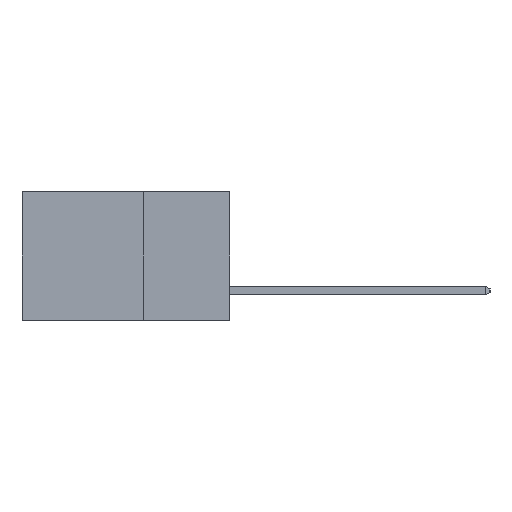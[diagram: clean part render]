
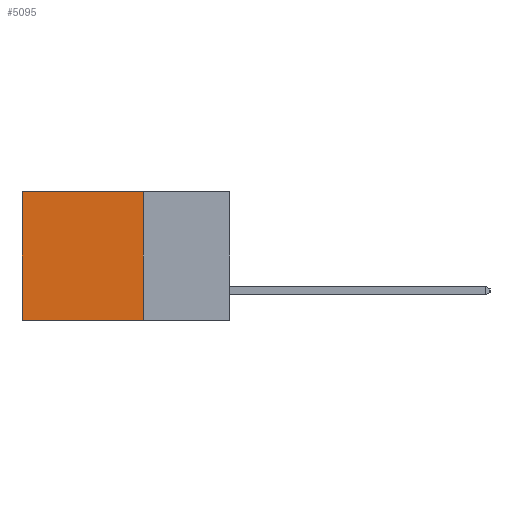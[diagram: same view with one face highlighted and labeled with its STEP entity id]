
A CAD part, left-side view. The second image highlights one B-rep face of the part: STEP entity #5095.
In plain terms, the highlighted planar face has unit normal (-1, 0, 0).
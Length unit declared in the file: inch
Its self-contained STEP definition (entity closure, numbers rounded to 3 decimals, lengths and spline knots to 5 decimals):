
#164 = DIRECTION ( 'NONE',  ( 0., 0., -1. ) ) ;
#1007 = CARTESIAN_POINT ( 'NONE',  ( 0.298, 0.6, 0. ) ) ;
#1571 = EDGE_CURVE ( 'NONE', #13154, #3747, #12394, .T. ) ;
#2009 = CARTESIAN_POINT ( 'NONE',  ( 0.298, 0.25, 0. ) ) ;
#2358 = PLANE ( 'NONE',  #6312 ) ;
#2890 = VECTOR ( 'NONE', #164, 39.37008 ) ;
#3245 = DIRECTION ( 'NONE',  ( 1., 0., 0. ) ) ;
#3601 = LINE ( 'NONE', #6369, #11280 ) ;
#3747 = VERTEX_POINT ( 'NONE', #11857 ) ;
#4230 = DIRECTION ( 'NONE',  ( 0., 0., -1. ) ) ;
#4520 = LINE ( 'NONE', #11120, #12372 ) ;
#4640 = ORIENTED_EDGE ( 'NONE', *, *, #1571, .T. ) ;
#4713 = ORIENTED_EDGE ( 'NONE', *, *, #4885, .F. ) ;
#4726 = ORIENTED_EDGE ( 'NONE', *, *, #7457, .F. ) ;
#4738 = ORIENTED_EDGE ( 'NONE', *, *, #6700, .T. ) ;
#4885 = EDGE_CURVE ( 'NONE', #10407, #3747, #4520, .T. ) ;
#5095 = ADVANCED_FACE ( 'NONE', ( #11925 ), #2358, .F. ) ;
#5804 = LINE ( 'NONE', #10744, #2890 ) ;
#6312 = AXIS2_PLACEMENT_3D ( 'NONE', #2009, #3245, #4230 ) ;
#6369 = CARTESIAN_POINT ( 'NONE',  ( 0.298, 0.25, 0. ) ) ;
#6700 = EDGE_CURVE ( 'NONE', #13024, #13154, #3601, .T. ) ;
#7457 = EDGE_CURVE ( 'NONE', #13024, #10407, #5804, .T. ) ;
#7607 = DIRECTION ( 'NONE',  ( 0., 1., 0. ) ) ;
#9096 = CARTESIAN_POINT ( 'NONE',  ( 0.298, 0.25, 0. ) ) ;
#9498 = DIRECTION ( 'NONE',  ( 0., 0., -1. ) ) ;
#9677 = CARTESIAN_POINT ( 'NONE',  ( 0.298, 0.6, 0. ) ) ;
#10407 = VERTEX_POINT ( 'NONE', #12334 ) ;
#10437 = DIRECTION ( 'NONE',  ( 0., 1., 0. ) ) ;
#10744 = CARTESIAN_POINT ( 'NONE',  ( 0.298, 0.25, 0. ) ) ;
#11120 = CARTESIAN_POINT ( 'NONE',  ( 0.298, 0.25, -0.37 ) ) ;
#11146 = EDGE_LOOP ( 'NONE', ( #4640, #4713, #4726, #4738 ) ) ;
#11280 = VECTOR ( 'NONE', #10437, 39.37008 ) ;
#11857 = CARTESIAN_POINT ( 'NONE',  ( 0.298, 0.6, -0.37 ) ) ;
#11925 = FACE_OUTER_BOUND ( 'NONE', #11146, .T. ) ;
#12099 = VECTOR ( 'NONE', #9498, 39.37008 ) ;
#12334 = CARTESIAN_POINT ( 'NONE',  ( 0.298, 0.25, -0.37 ) ) ;
#12372 = VECTOR ( 'NONE', #7607, 39.37008 ) ;
#12394 = LINE ( 'NONE', #9677, #12099 ) ;
#13024 = VERTEX_POINT ( 'NONE', #9096 ) ;
#13154 = VERTEX_POINT ( 'NONE', #1007 ) ;
